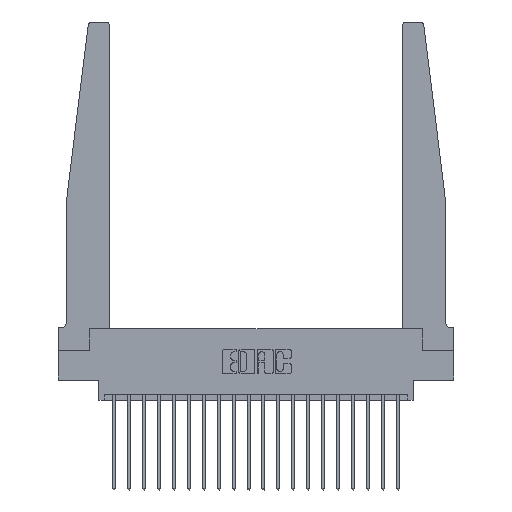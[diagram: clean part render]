
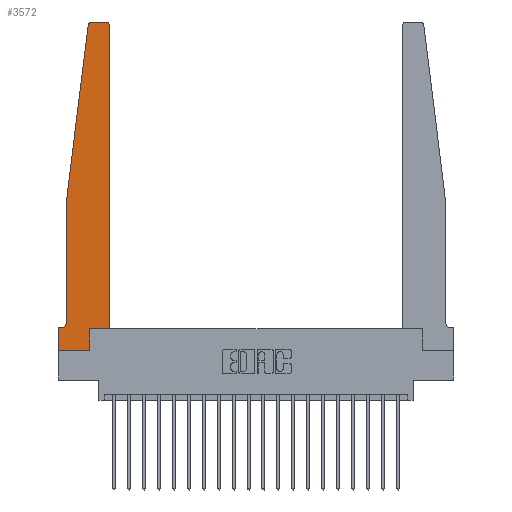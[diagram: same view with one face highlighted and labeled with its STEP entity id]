
A CAD part, top view. The second image highlights one B-rep face of the part: STEP entity #3572.
In plain terms, the highlighted planar face has unit normal (0, 0, 1).
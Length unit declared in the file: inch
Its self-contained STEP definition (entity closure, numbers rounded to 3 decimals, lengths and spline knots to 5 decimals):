
#289 = CARTESIAN_POINT ( 'NONE',  ( 0.015, 0.1875, 0.37 ) ) ;
#301 = VERTEX_POINT ( 'NONE', #1788 ) ;
#502 = DIRECTION ( 'NONE',  ( 0., -1., 0. ) ) ;
#583 = ORIENTED_EDGE ( 'NONE', *, *, #6163, .T. ) ;
#721 = LINE ( 'NONE', #7307, #13178 ) ;
#869 = DIRECTION ( 'NONE',  ( -1., 0., 0. ) ) ;
#931 = CARTESIAN_POINT ( 'NONE',  ( 0.425, 0.18, 0.37 ) ) ;
#1024 = ORIENTED_EDGE ( 'NONE', *, *, #1101, .T. ) ;
#1101 = EDGE_CURVE ( 'NONE', #20039, #16971, #17344, .T. ) ;
#1133 = CIRCLE ( 'NONE', #7332, 0.03 ) ;
#1240 = VERTEX_POINT ( 'NONE', #6592 ) ;
#1249 = ORIENTED_EDGE ( 'NONE', *, *, #5237, .T. ) ;
#1562 = CARTESIAN_POINT ( 'NONE',  ( 0.27653, 2.75, 0.37 ) ) ;
#1788 = CARTESIAN_POINT ( 'NONE',  ( 0.2605, 0.18, 0.37 ) ) ;
#1962 = EDGE_LOOP ( 'NONE', ( #14432, #12941, #9777, #1249, #7851, #1024, #14263, #2145, #19750, #19570, #583, #4281 ) ) ;
#1988 = DIRECTION ( 'NONE',  ( -1., 0., 0. ) ) ;
#2130 = CARTESIAN_POINT ( 'NONE',  ( 0.425, 0.18, 0.37 ) ) ;
#2145 = ORIENTED_EDGE ( 'NONE', *, *, #11942, .T. ) ;
#2441 = DIRECTION ( 'NONE',  ( 1., 0., 0. ) ) ;
#2512 = CARTESIAN_POINT ( 'NONE',  ( 0.065, 1.25, 0.37 ) ) ;
#2809 = DIRECTION ( 'NONE',  ( 1., 0., 0. ) ) ;
#3168 = LINE ( 'NONE', #3488, #11555 ) ;
#3319 = LINE ( 'NONE', #8295, #13669 ) ;
#3328 = EDGE_CURVE ( 'NONE', #7947, #20167, #1133, .T. ) ;
#3488 = CARTESIAN_POINT ( 'NONE',  ( 0., 0., 0.37 ) ) ;
#3572 = ADVANCED_FACE ( 'NONE', ( #6866 ), #20096, .T. ) ;
#4053 = VECTOR ( 'NONE', #7314, 39.37008 ) ;
#4223 = CARTESIAN_POINT ( 'NONE',  ( 0.065, 1.25, 0.37 ) ) ;
#4254 = LINE ( 'NONE', #13804, #5407 ) ;
#4281 = ORIENTED_EDGE ( 'NONE', *, *, #11033, .T. ) ;
#5237 = EDGE_CURVE ( 'NONE', #10585, #1240, #7729, .T. ) ;
#5407 = VECTOR ( 'NONE', #502, 39.37008 ) ;
#5562 = EDGE_CURVE ( 'NONE', #20167, #10585, #7369, .T. ) ;
#6008 = DIRECTION ( 'NONE',  ( 0., -1., 0. ) ) ;
#6163 = EDGE_CURVE ( 'NONE', #17379, #18214, #721, .T. ) ;
#6592 = CARTESIAN_POINT ( 'NONE',  ( 0.065, 0.2375, 0.37 ) ) ;
#6751 = AXIS2_PLACEMENT_3D ( 'NONE', #15233, #18361, #10002 ) ;
#6866 = FACE_OUTER_BOUND ( 'NONE', #1962, .T. ) ;
#7232 = CARTESIAN_POINT ( 'NONE',  ( 0.015, 0.2375, 0.37 ) ) ;
#7307 = CARTESIAN_POINT ( 'NONE',  ( 0.425, 0.18, 0.37 ) ) ;
#7314 = DIRECTION ( 'NONE',  ( 1., 0., 0. ) ) ;
#7332 = AXIS2_PLACEMENT_3D ( 'NONE', #9135, #7420, #2441 ) ;
#7369 = LINE ( 'NONE', #4223, #12687 ) ;
#7420 = DIRECTION ( 'NONE',  ( 0., 0., 1. ) ) ;
#7432 = VERTEX_POINT ( 'NONE', #16652 ) ;
#7505 = VERTEX_POINT ( 'NONE', #11521 ) ;
#7612 = EDGE_CURVE ( 'NONE', #16971, #7505, #4254, .T. ) ;
#7729 = LINE ( 'NONE', #10861, #10887 ) ;
#7851 = ORIENTED_EDGE ( 'NONE', *, *, #14742, .T. ) ;
#7947 = VERTEX_POINT ( 'NONE', #1562 ) ;
#8295 = CARTESIAN_POINT ( 'NONE',  ( 0.2605, 0.18, 0.37 ) ) ;
#9135 = CARTESIAN_POINT ( 'NONE',  ( 0.27653, 2.72, 0.37 ) ) ;
#9460 = EDGE_CURVE ( 'NONE', #21131, #7947, #16842, .T. ) ;
#9777 = ORIENTED_EDGE ( 'NONE', *, *, #5562, .T. ) ;
#10002 = DIRECTION ( 'NONE',  ( 1., 0., 0. ) ) ;
#10143 = AXIS2_PLACEMENT_3D ( 'NONE', #10702, #17341, #2809 ) ;
#10361 = DIRECTION ( 'NONE',  ( -1., 0., 0. ) ) ;
#10585 = VERTEX_POINT ( 'NONE', #2512 ) ;
#10702 = CARTESIAN_POINT ( 'NONE',  ( 0.395, 2.72, 0.37 ) ) ;
#10812 = DIRECTION ( 'NONE',  ( -0.122, -0.992, 0. ) ) ;
#10861 = CARTESIAN_POINT ( 'NONE',  ( 0.065, 1.25, 0.37 ) ) ;
#10887 = VECTOR ( 'NONE', #6008, 39.37008 ) ;
#11033 = EDGE_CURVE ( 'NONE', #18214, #21131, #11859, .T. ) ;
#11521 = CARTESIAN_POINT ( 'NONE',  ( 0., 0., 0.37 ) ) ;
#11555 = VECTOR ( 'NONE', #16617, 39.37008 ) ;
#11859 = CIRCLE ( 'NONE', #10143, 0.03 ) ;
#11871 = DIRECTION ( 'NONE',  ( 0., 0., -1. ) ) ;
#11942 = EDGE_CURVE ( 'NONE', #7505, #7432, #3168, .T. ) ;
#12687 = VECTOR ( 'NONE', #10812, 39.37008 ) ;
#12941 = ORIENTED_EDGE ( 'NONE', *, *, #3328, .T. ) ;
#13178 = VECTOR ( 'NONE', #14019, 39.37008 ) ;
#13525 = CARTESIAN_POINT ( 'NONE',  ( 0., 0.1875, 0.37 ) ) ;
#13669 = VECTOR ( 'NONE', #16438, 39.37008 ) ;
#13804 = CARTESIAN_POINT ( 'NONE',  ( 0., 0., 0.37 ) ) ;
#14019 = DIRECTION ( 'NONE',  ( 0., 1., 0. ) ) ;
#14263 = ORIENTED_EDGE ( 'NONE', *, *, #7612, .T. ) ;
#14432 = ORIENTED_EDGE ( 'NONE', *, *, #9460, .T. ) ;
#14712 = AXIS2_PLACEMENT_3D ( 'NONE', #7232, #11871, #10361 ) ;
#14742 = EDGE_CURVE ( 'NONE', #1240, #20039, #21283, .T. ) ;
#14935 = CARTESIAN_POINT ( 'NONE',  ( 0.425, 2.72, 0.37 ) ) ;
#14977 = EDGE_CURVE ( 'NONE', #7432, #301, #3319, .T. ) ;
#15233 = CARTESIAN_POINT ( 'NONE',  ( 0., 0.1875, 0.37 ) ) ;
#16077 = CARTESIAN_POINT ( 'NONE',  ( 0.24675, 2.72367, 0.37 ) ) ;
#16438 = DIRECTION ( 'NONE',  ( 0., 1., 0. ) ) ;
#16617 = DIRECTION ( 'NONE',  ( 1., 0., 0. ) ) ;
#16652 = CARTESIAN_POINT ( 'NONE',  ( 0.2605, 0., 0.37 ) ) ;
#16842 = LINE ( 'NONE', #19571, #17031 ) ;
#16971 = VERTEX_POINT ( 'NONE', #13525 ) ;
#16979 = LINE ( 'NONE', #2130, #4053 ) ;
#17031 = VECTOR ( 'NONE', #1988, 39.37008 ) ;
#17333 = EDGE_CURVE ( 'NONE', #301, #17379, #16979, .T. ) ;
#17341 = DIRECTION ( 'NONE',  ( 0., 0., 1. ) ) ;
#17344 = LINE ( 'NONE', #17445, #19307 ) ;
#17379 = VERTEX_POINT ( 'NONE', #931 ) ;
#17445 = CARTESIAN_POINT ( 'NONE',  ( 0.065, 0.1875, 0.37 ) ) ;
#18214 = VERTEX_POINT ( 'NONE', #14935 ) ;
#18361 = DIRECTION ( 'NONE',  ( 0., 0., 1. ) ) ;
#19307 = VECTOR ( 'NONE', #869, 39.37008 ) ;
#19570 = ORIENTED_EDGE ( 'NONE', *, *, #17333, .T. ) ;
#19571 = CARTESIAN_POINT ( 'NONE',  ( 0.25, 2.75, 0.37 ) ) ;
#19750 = ORIENTED_EDGE ( 'NONE', *, *, #14977, .T. ) ;
#20039 = VERTEX_POINT ( 'NONE', #289 ) ;
#20096 = PLANE ( 'NONE',  #6751 ) ;
#20167 = VERTEX_POINT ( 'NONE', #16077 ) ;
#20894 = CARTESIAN_POINT ( 'NONE',  ( 0.395, 2.75, 0.37 ) ) ;
#21131 = VERTEX_POINT ( 'NONE', #20894 ) ;
#21283 = CIRCLE ( 'NONE', #14712, 0.05 ) ;
